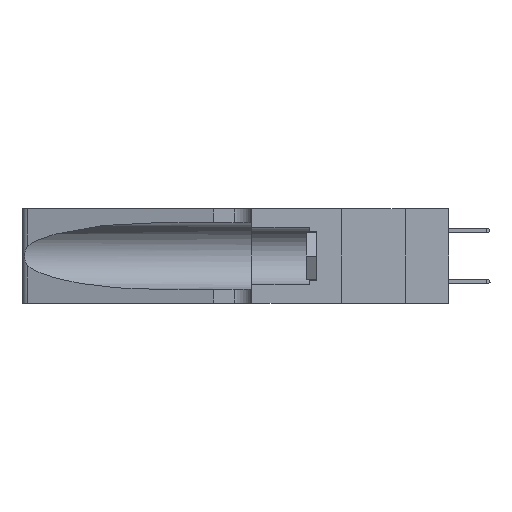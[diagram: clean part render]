
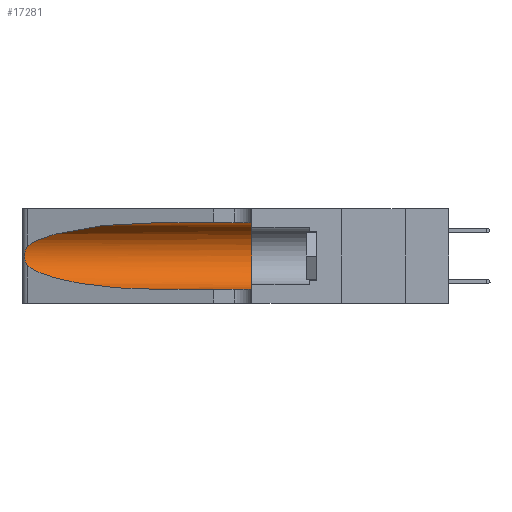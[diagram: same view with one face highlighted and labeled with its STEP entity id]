
A CAD part, left-side view. The second image highlights one B-rep face of the part: STEP entity #17281.
In plain terms, the highlighted cylindrical face has radius 3.308 mm (diameter 6.617 mm), a partial arc.
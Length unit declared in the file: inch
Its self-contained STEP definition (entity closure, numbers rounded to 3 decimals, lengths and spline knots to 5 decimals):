
#505 = B_SPLINE_CURVE_WITH_KNOTS ( 'NONE', 3,
 ( #2781, #2491, #5163, #7503, #23742, #9834, #7298, #11865, #523, #5265, #4867, #23436, #19615, #28619 ),
 .UNSPECIFIED., .F., .F.,
 ( 4, 2, 2, 2, 2, 2, 4 ),
 ( 0., 0.00027, 0.00053, 0.00107, 0.0016, 0.00187, 0.00214 ),
 .UNSPECIFIED. ) ;
#523 = CARTESIAN_POINT ( 'NONE',  ( 0.26017, 1.23833, 0.17102 ) ) ;
#720 = DIRECTION ( 'NONE',  ( 0., -1., 0. ) ) ;
#791 = AXIS2_PLACEMENT_3D ( 'NONE', #22214, #24239, #26691 ) ;
#1167 = ORIENTED_EDGE ( 'NONE', *, *, #11769, .F. ) ;
#1950 = CARTESIAN_POINT ( 'NONE',  ( 0.1305, 0.35, 0.31525 ) ) ;
#1982 = CARTESIAN_POINT ( 'NONE',  ( 0.2373, 1.15595, 0.08982 ) ) ;
#2491 = CARTESIAN_POINT ( 'NONE',  ( 0.25555, 1.22994, 0.2215 ) ) ;
#2723 = FACE_OUTER_BOUND ( 'NONE', #12465, .T. ) ;
#2781 = CARTESIAN_POINT ( 'NONE',  ( 0.25487, 1.22718, 0.22369 ) ) ;
#3208 = CARTESIAN_POINT ( 'NONE',  ( 0.1305, 1.61858, 0.31525 ) ) ;
#3372 = EDGE_CURVE ( 'NONE', #4169, #11774, #12970, .T. ) ;
#3425 = LINE ( 'NONE', #3208, #17243 ) ;
#3851 = ORIENTED_EDGE ( 'NONE', *, *, #9949, .T. ) ;
#4169 = VERTEX_POINT ( 'NONE', #1950 ) ;
#4522 = CARTESIAN_POINT ( 'NONE',  ( 0.18966, 0.96281, 0.05475 ) ) ;
#4867 = CARTESIAN_POINT ( 'NONE',  ( 0.25789, 1.23486, 0.15765 ) ) ;
#5163 = CARTESIAN_POINT ( 'NONE',  ( 0.25639, 1.23184, 0.21858 ) ) ;
#5265 = CARTESIAN_POINT ( 'NONE',  ( 0.25856, 1.23593, 0.16098 ) ) ;
#7298 = CARTESIAN_POINT ( 'NONE',  ( 0.26075, 1.23896, 0.19203 ) ) ;
#7503 = CARTESIAN_POINT ( 'NONE',  ( 0.25787, 1.23484, 0.2124 ) ) ;
#7789 = CARTESIAN_POINT ( 'NONE',  ( 0.1305, 1.61858, 0.185 ) ) ;
#8265 = CYLINDRICAL_SURFACE ( 'NONE', #16784, 0.13025 ) ;
#8540 = VERTEX_POINT ( 'NONE', #19880 ) ;
#9233 = CARTESIAN_POINT ( 'NONE',  ( 0.1305, 0.72297, 0.05475 ) ) ;
#9779 = EDGE_CURVE ( 'NONE', #18828, #11774, #26796, .T. ) ;
#9834 = CARTESIAN_POINT ( 'NONE',  ( 0.26018, 1.23835, 0.19895 ) ) ;
#9949 = EDGE_CURVE ( 'NONE', #8540, #21761, #505, .T. ) ;
#10034 = VERTEX_POINT ( 'NONE', #25314 ) ;
#11599 = DIRECTION ( 'NONE',  ( 0., -1., 0. ) ) ;
#11769 = EDGE_CURVE ( 'NONE', #10034, #4169, #3425, .T. ) ;
#11774 = VERTEX_POINT ( 'NONE', #22322 ) ;
#11865 = CARTESIAN_POINT ( 'NONE',  ( 0.26075, 1.23896, 0.178 ) ) ;
#12465 = EDGE_LOOP ( 'NONE', ( #16431, #3851, #18976, #26757, #26567, #1167 ) ) ;
#12970 = CIRCLE ( 'NONE', #791, 0.13025 ) ;
#13964 = EDGE_CURVE ( 'NONE', #21761, #18828, #28502, .T. ) ;
#14306 = CARTESIAN_POINT ( 'NONE',  ( 0.25487, 1.22718, 0.14631 ) ) ;
#14772 = VECTOR ( 'NONE', #11599, 39.37008 ) ;
#14924 = CARTESIAN_POINT ( 'NONE',  ( 0.2373, 1.15595, 0.28018 ) ) ;
#15919 = CARTESIAN_POINT ( 'NONE',  ( 0.25487, 1.22718, 0.14631 ) ) ;
#16431 = ORIENTED_EDGE ( 'NONE', *, *, #26974, .T. ) ;
#16784 = AXIS2_PLACEMENT_3D ( 'NONE', #7789, #720, #26679 ) ;
#17225 = DIRECTION ( 'NONE',  ( 0., -1., 0. ) ) ;
#17243 = VECTOR ( 'NONE', #17225, 39.37008 ) ;
#17281 = ADVANCED_FACE ( 'NONE', ( #2723 ), #8265, .F. ) ;
#18279 = CARTESIAN_POINT ( 'NONE',  ( 0.1305, 0.72297, 0.05475 ) ) ;
#18828 = VERTEX_POINT ( 'NONE', #18279 ) ;
#18976 = ORIENTED_EDGE ( 'NONE', *, *, #13964, .T. ) ;
#19615 = CARTESIAN_POINT ( 'NONE',  ( 0.25555, 1.22993, 0.14849 ) ) ;
#19880 = CARTESIAN_POINT ( 'NONE',  ( 0.25487, 1.22718, 0.22369 ) ) ;
#21761 = VERTEX_POINT ( 'NONE', #14306 ) ;
#21825 = CARTESIAN_POINT ( 'NONE',  ( 0.18966, 0.96281, 0.31525 ) ) ;
#21932 = CARTESIAN_POINT ( 'NONE',  ( 0.25487, 1.22718, 0.22369 ) ) ;
#22139 = CARTESIAN_POINT ( 'NONE',  ( 0.1305, 0.72297, 0.31525 ) ) ;
#22214 = CARTESIAN_POINT ( 'NONE',  ( 0.1305, 0.35, 0.185 ) ) ;
#22322 = CARTESIAN_POINT ( 'NONE',  ( 0.1305, 0.35, 0.05475 ) ) ;
#23080 = CARTESIAN_POINT ( 'NONE',  ( 0.1305, 1.61858, 0.05475 ) ) ;
#23436 = CARTESIAN_POINT ( 'NONE',  ( 0.25639, 1.23186, 0.15144 ) ) ;
#23742 = CARTESIAN_POINT ( 'NONE',  ( 0.25854, 1.2359, 0.20912 ) ) ;
#24239 = DIRECTION ( 'NONE',  ( 0., 1., 0. ) ) ;
#25314 = CARTESIAN_POINT ( 'NONE',  ( 0.1305, 0.72297, 0.31525 ) ) ;
#26260 =( BOUNDED_CURVE ( )  B_SPLINE_CURVE ( 3, ( #22139, #21825, #14924, #21932 ),
 .UNSPECIFIED., .F., .T. ) 
 B_SPLINE_CURVE_WITH_KNOTS ( ( 4, 4 ),
 ( 1.5708, 2.84003 ),
 .UNSPECIFIED. ) 
 CURVE ( )  GEOMETRIC_REPRESENTATION_ITEM ( )  RATIONAL_B_SPLINE_CURVE ( ( 1., 0.87, 0.87, 1. ) ) 
 REPRESENTATION_ITEM ( '' )  );
#26567 = ORIENTED_EDGE ( 'NONE', *, *, #3372, .F. ) ;
#26679 = DIRECTION ( 'NONE',  ( 0., 0., -1. ) ) ;
#26691 = DIRECTION ( 'NONE',  ( 0., 0., 1. ) ) ;
#26757 = ORIENTED_EDGE ( 'NONE', *, *, #9779, .T. ) ;
#26796 = LINE ( 'NONE', #23080, #14772 ) ;
#26974 = EDGE_CURVE ( 'NONE', #10034, #8540, #26260, .T. ) ;
#28502 =( BOUNDED_CURVE ( )  B_SPLINE_CURVE ( 3, ( #15919, #1982, #4522, #9233 ),
 .UNSPECIFIED., .F., .F. ) 
 B_SPLINE_CURVE_WITH_KNOTS ( ( 4, 4 ),
 ( 3.44316, 4.71239 ),
 .UNSPECIFIED. ) 
 CURVE ( )  GEOMETRIC_REPRESENTATION_ITEM ( )  RATIONAL_B_SPLINE_CURVE ( ( 1., 0.87, 0.87, 1. ) ) 
 REPRESENTATION_ITEM ( '' )  );
#28619 = CARTESIAN_POINT ( 'NONE',  ( 0.25487, 1.22718, 0.14631 ) ) ;
